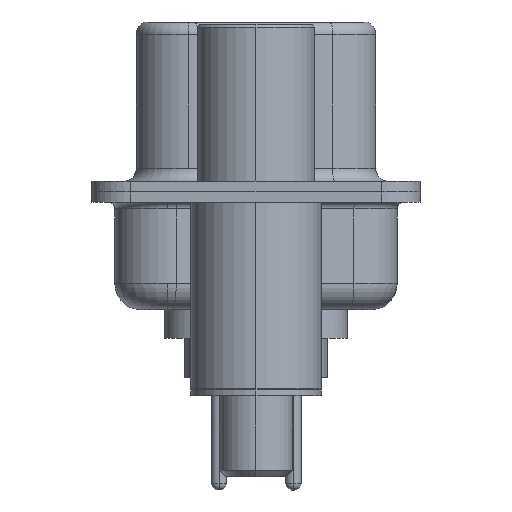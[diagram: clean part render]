
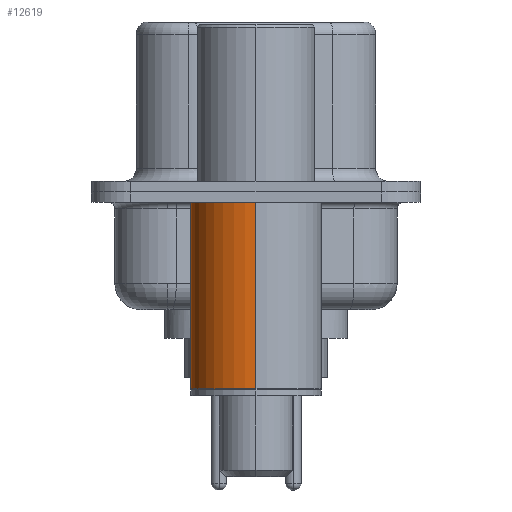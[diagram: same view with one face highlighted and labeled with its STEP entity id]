
A CAD part, left-side view. The second image highlights one B-rep face of the part: STEP entity #12619.
In plain terms, the highlighted cylindrical face has radius 2.5 mm (diameter 5 mm), a partial arc.
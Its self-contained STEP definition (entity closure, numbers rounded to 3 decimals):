
#838 = LINE ( 'NONE', #6843, #6280 ) ;
#1761 = AXIS2_PLACEMENT_3D ( 'NONE', #1818, #9848, #1911 ) ;
#1818 = CARTESIAN_POINT ( 'NONE',  ( 0., 0., -7.525 ) ) ;
#1911 = DIRECTION ( 'NONE',  ( 1., 0., 0. ) ) ;
#2671 = CARTESIAN_POINT ( 'NONE',  ( -2.5, 0., -0.4 ) ) ;
#3261 = DIRECTION ( 'NONE',  ( 0., 0., 1. ) ) ;
#3410 = VERTEX_POINT ( 'NONE', #2671 ) ;
#3589 = CARTESIAN_POINT ( 'NONE',  ( 0., 0., 0.581 ) ) ;
#4172 = CIRCLE ( 'NONE', #1761, 2.5 ) ;
#4886 = EDGE_LOOP ( 'NONE', ( #15853, #25972, #9629, #22946 ) ) ;
#5406 = VECTOR ( 'NONE', #3261, 1000. ) ;
#6280 = VECTOR ( 'NONE', #25009, 1000. ) ;
#6305 = VERTEX_POINT ( 'NONE', #20534 ) ;
#6620 = AXIS2_PLACEMENT_3D ( 'NONE', #15262, #21807, #21723 ) ;
#6843 = CARTESIAN_POINT ( 'NONE',  ( -2.5, 0., 0.581 ) ) ;
#7358 = EDGE_CURVE ( 'NONE', #6305, #3410, #838, .T. ) ;
#8787 = VERTEX_POINT ( 'NONE', #13871 ) ;
#9629 = ORIENTED_EDGE ( 'NONE', *, *, #16066, .F. ) ;
#9807 = DIRECTION ( 'NONE',  ( 0., 0., 1. ) ) ;
#9848 = DIRECTION ( 'NONE',  ( 0., 0., 1. ) ) ;
#11761 = DIRECTION ( 'NONE',  ( 1., 0., 0. ) ) ;
#12619 = ADVANCED_FACE ( 'NONE', ( #20553 ), #18311, .T. ) ;
#12719 = CIRCLE ( 'NONE', #6620, 2.5 ) ;
#13871 = CARTESIAN_POINT ( 'NONE',  ( 2.5, 0., -7.525 ) ) ;
#14465 = VERTEX_POINT ( 'NONE', #17187 ) ;
#14849 = EDGE_CURVE ( 'NONE', #8787, #14465, #17537, .T. ) ;
#15262 = CARTESIAN_POINT ( 'NONE',  ( 0., 0., -0.4 ) ) ;
#15853 = ORIENTED_EDGE ( 'NONE', *, *, #26511, .T. ) ;
#16066 = EDGE_CURVE ( 'NONE', #14465, #3410, #12719, .T. ) ;
#17187 = CARTESIAN_POINT ( 'NONE',  ( 2.5, 0., -0.4 ) ) ;
#17537 = LINE ( 'NONE', #19470, #5406 ) ;
#18311 = CYLINDRICAL_SURFACE ( 'NONE', #24336, 2.5 ) ;
#19470 = CARTESIAN_POINT ( 'NONE',  ( 2.5, 0., 0.581 ) ) ;
#20534 = CARTESIAN_POINT ( 'NONE',  ( -2.5, 0., -7.525 ) ) ;
#20553 = FACE_OUTER_BOUND ( 'NONE', #4886, .T. ) ;
#21723 = DIRECTION ( 'NONE',  ( 1., 0., 0. ) ) ;
#21807 = DIRECTION ( 'NONE',  ( 0., 0., 1. ) ) ;
#22946 = ORIENTED_EDGE ( 'NONE', *, *, #14849, .F. ) ;
#24336 = AXIS2_PLACEMENT_3D ( 'NONE', #3589, #9807, #11761 ) ;
#25009 = DIRECTION ( 'NONE',  ( 0., 0., 1. ) ) ;
#25972 = ORIENTED_EDGE ( 'NONE', *, *, #7358, .T. ) ;
#26511 = EDGE_CURVE ( 'NONE', #8787, #6305, #4172, .T. ) ;
